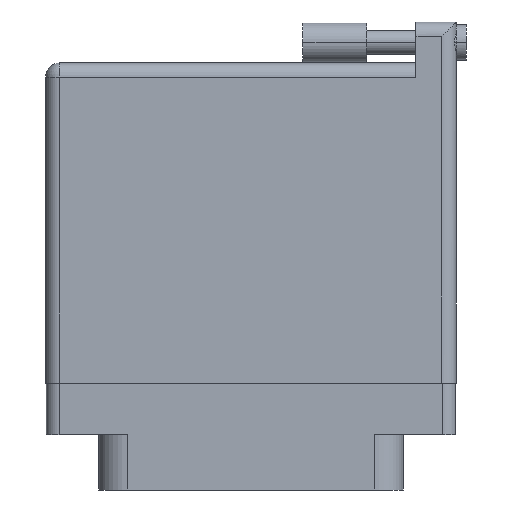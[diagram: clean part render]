
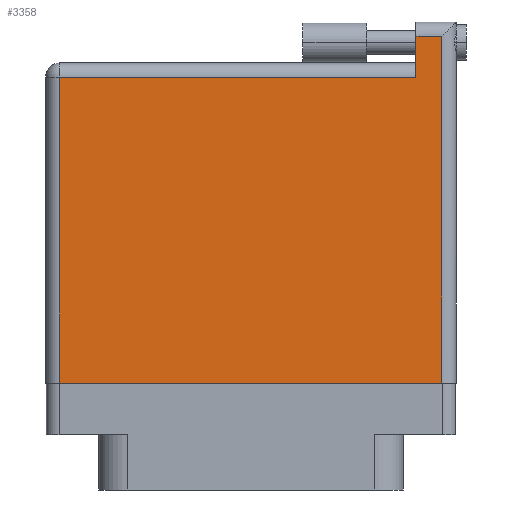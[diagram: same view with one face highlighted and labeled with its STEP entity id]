
A CAD part, front view. The second image highlights one B-rep face of the part: STEP entity #3358.
In plain terms, the highlighted face is planar.
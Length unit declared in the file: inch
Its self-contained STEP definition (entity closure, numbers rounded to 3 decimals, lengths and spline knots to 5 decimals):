
#877 = LINE ( 'NONE', #12085, #34685 ) ;
#997 = CARTESIAN_POINT ( 'NONE',  ( 0.934, -0.1, 0.4495 ) ) ;
#1249 = PLANE ( 'NONE',  #8776 ) ;
#1911 = CARTESIAN_POINT ( 'NONE',  ( 0.807, 1.666, 0.4495 ) ) ;
#2253 = ORIENTED_EDGE ( 'NONE', *, *, #32139, .T. ) ;
#2921 = ORIENTED_EDGE ( 'NONE', *, *, #25666, .T. ) ;
#2960 = ORIENTED_EDGE ( 'NONE', *, *, #26297, .T. ) ;
#3358 = ADVANCED_FACE ( 'NONE', ( #29165 ), #1249, .F. ) ;
#4328 = DIRECTION ( 'NONE',  ( 0., 0., -1. ) ) ;
#4749 = DIRECTION ( 'NONE',  ( 0., -1., 0. ) ) ;
#5380 = VERTEX_POINT ( 'NONE', #9668 ) ;
#6137 = DIRECTION ( 'NONE',  ( -1., 0., 0. ) ) ;
#7254 = ORIENTED_EDGE ( 'NONE', *, *, #16777, .T. ) ;
#7330 = LINE ( 'NONE', #20933, #22897 ) ;
#7444 = EDGE_CURVE ( 'NONE', #28150, #15839, #33435, .T. ) ;
#8389 = DIRECTION ( 'NONE',  ( 1., 0., 0. ) ) ;
#8571 = DIRECTION ( 'NONE',  ( 0., 1., 0. ) ) ;
#8776 = AXIS2_PLACEMENT_3D ( 'NONE', #12289, #4328, #26443 ) ;
#9668 = CARTESIAN_POINT ( 'NONE',  ( -0.934, 1.396, 0.4495 ) ) ;
#10412 = LINE ( 'NONE', #1911, #12196 ) ;
#11852 = CARTESIAN_POINT ( 'NONE',  ( 0.934, 1.596, 0.4495 ) ) ;
#12085 = CARTESIAN_POINT ( 'NONE',  ( -1.004, 1.596, 0.4495 ) ) ;
#12196 = VECTOR ( 'NONE', #35098, 39.37008 ) ;
#12289 = CARTESIAN_POINT ( 'NONE',  ( -1.004, 1.466, 0.4495 ) ) ;
#13174 = VERTEX_POINT ( 'NONE', #27046 ) ;
#14359 = CARTESIAN_POINT ( 'NONE',  ( -1.004, -0.1, 0.4495 ) ) ;
#15195 = CARTESIAN_POINT ( 'NONE',  ( 0.807, 1.396, 0.4495 ) ) ;
#15839 = VERTEX_POINT ( 'NONE', #11852 ) ;
#16316 = LINE ( 'NONE', #27409, #26513 ) ;
#16777 = EDGE_CURVE ( 'NONE', #13174, #30996, #10412, .T. ) ;
#18831 = EDGE_LOOP ( 'NONE', ( #2253, #27633, #2960, #7254, #22109, #2921 ) ) ;
#19279 = VECTOR ( 'NONE', #8389, 39.37008 ) ;
#20933 = CARTESIAN_POINT ( 'NONE',  ( -1.004, 1.396, 0.4495 ) ) ;
#21148 = CARTESIAN_POINT ( 'NONE',  ( -0.934, -0.1, 0.4495 ) ) ;
#21478 = EDGE_CURVE ( 'NONE', #30996, #5380, #7330, .T. ) ;
#21712 = VECTOR ( 'NONE', #8571, 39.37008 ) ;
#22109 = ORIENTED_EDGE ( 'NONE', *, *, #21478, .T. ) ;
#22897 = VECTOR ( 'NONE', #32014, 39.37008 ) ;
#25407 = LINE ( 'NONE', #14359, #19279 ) ;
#25666 = EDGE_CURVE ( 'NONE', #5380, #26453, #16316, .T. ) ;
#26297 = EDGE_CURVE ( 'NONE', #15839, #13174, #877, .T. ) ;
#26443 = DIRECTION ( 'NONE',  ( -1., 0., 0. ) ) ;
#26453 = VERTEX_POINT ( 'NONE', #21148 ) ;
#26513 = VECTOR ( 'NONE', #4749, 39.37008 ) ;
#27046 = CARTESIAN_POINT ( 'NONE',  ( 0.807, 1.596, 0.4495 ) ) ;
#27409 = CARTESIAN_POINT ( 'NONE',  ( -0.934, -0.1, 0.4495 ) ) ;
#27633 = ORIENTED_EDGE ( 'NONE', *, *, #7444, .T. ) ;
#28150 = VERTEX_POINT ( 'NONE', #997 ) ;
#29165 = FACE_OUTER_BOUND ( 'NONE', #18831, .T. ) ;
#30996 = VERTEX_POINT ( 'NONE', #15195 ) ;
#32014 = DIRECTION ( 'NONE',  ( -1., 0., 0. ) ) ;
#32139 = EDGE_CURVE ( 'NONE', #26453, #28150, #25407, .T. ) ;
#33435 = LINE ( 'NONE', #35599, #21712 ) ;
#34685 = VECTOR ( 'NONE', #6137, 39.37008 ) ;
#35098 = DIRECTION ( 'NONE',  ( 0., -1., 0. ) ) ;
#35599 = CARTESIAN_POINT ( 'NONE',  ( 0.934, 1.666, 0.4495 ) ) ;
